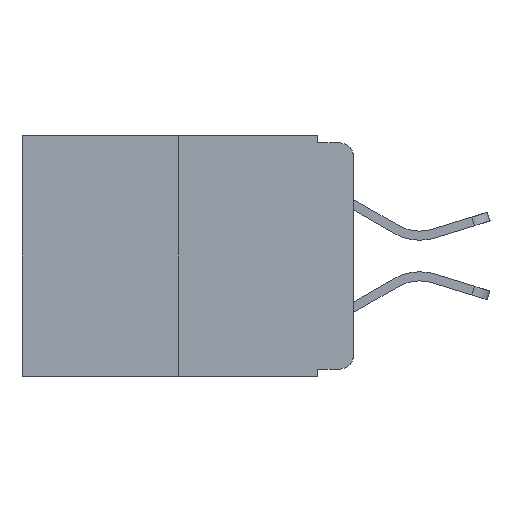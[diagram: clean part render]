
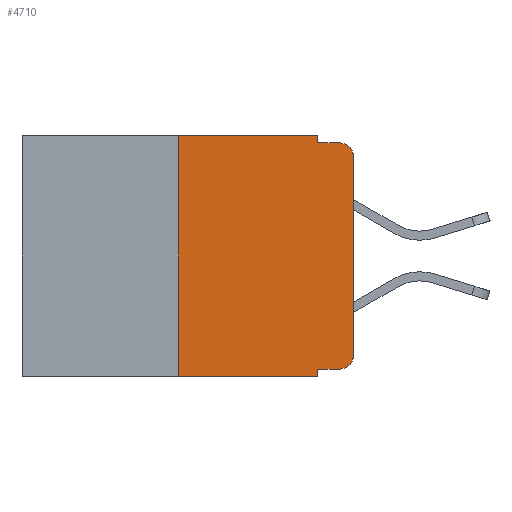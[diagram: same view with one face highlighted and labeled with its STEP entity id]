
A CAD part, left-side view. The second image highlights one B-rep face of the part: STEP entity #4710.
In plain terms, the highlighted planar face has unit normal (-1, 0, 0).
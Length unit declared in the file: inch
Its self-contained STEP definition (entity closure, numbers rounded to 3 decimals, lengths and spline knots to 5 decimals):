
#582 = EDGE_CURVE ( 'NONE', #12568, #9888, #10768, .T. ) ;
#737 = ORIENTED_EDGE ( 'NONE', *, *, #1405, .T. ) ;
#827 = CARTESIAN_POINT ( 'NONE',  ( 0., 0.051, -0.01 ) ) ;
#965 = CARTESIAN_POINT ( 'NONE',  ( 0., 0.473, -0.343 ) ) ;
#1026 = VERTEX_POINT ( 'NONE', #8154 ) ;
#1145 = AXIS2_PLACEMENT_3D ( 'NONE', #11117, #4868, #12154 ) ;
#1344 = DIRECTION ( 'NONE',  ( 0., -1., 0. ) ) ;
#1399 = CARTESIAN_POINT ( 'NONE',  ( 0., 0.051, -0.343 ) ) ;
#1405 = EDGE_CURVE ( 'NONE', #1777, #12568, #5124, .T. ) ;
#1473 = ORIENTED_EDGE ( 'NONE', *, *, #10100, .F. ) ;
#1503 = CARTESIAN_POINT ( 'NONE',  ( 0., 0.25, 0. ) ) ;
#1566 = DIRECTION ( 'NONE',  ( 0., 0., -1. ) ) ;
#1664 = ORIENTED_EDGE ( 'NONE', *, *, #2156, .F. ) ;
#1777 = VERTEX_POINT ( 'NONE', #2124 ) ;
#1992 = LINE ( 'NONE', #965, #12823 ) ;
#2124 = CARTESIAN_POINT ( 'NONE',  ( 0., 0.051, -0.333 ) ) ;
#2156 = EDGE_CURVE ( 'NONE', #1777, #13808, #5975, .T. ) ;
#2220 = CARTESIAN_POINT ( 'NONE',  ( 0., 0.02, -0.03 ) ) ;
#2394 = DIRECTION ( 'NONE',  ( 0., -1., 0. ) ) ;
#2566 = CARTESIAN_POINT ( 'NONE',  ( 0., 0.051, 0. ) ) ;
#2843 = EDGE_CURVE ( 'NONE', #7511, #9590, #5285, .T. ) ;
#3279 = DIRECTION ( 'NONE',  ( 0., 0., -1. ) ) ;
#3535 = VECTOR ( 'NONE', #8475, 39.37008 ) ;
#3605 = EDGE_CURVE ( 'NONE', #10144, #8338, #6113, .T. ) ;
#3803 = AXIS2_PLACEMENT_3D ( 'NONE', #2220, #9687, #3279 ) ;
#3881 = ORIENTED_EDGE ( 'NONE', *, *, #582, .T. ) ;
#3937 = DIRECTION ( 'NONE',  ( 0., 0., 1. ) ) ;
#4086 = VECTOR ( 'NONE', #10811, 39.37008 ) ;
#4267 = CARTESIAN_POINT ( 'NONE',  ( 0., 0.02, -0.313 ) ) ;
#4328 = EDGE_CURVE ( 'NONE', #8338, #11201, #6434, .T. ) ;
#4508 = CARTESIAN_POINT ( 'NONE',  ( 0., 0., 0. ) ) ;
#4710 = ADVANCED_FACE ( 'NONE', ( #13141 ), #11159, .F. ) ;
#4717 = ORIENTED_EDGE ( 'NONE', *, *, #2843, .F. ) ;
#4794 = VECTOR ( 'NONE', #1344, 39.37008 ) ;
#4868 = DIRECTION ( 'NONE',  ( 1., 0., 0. ) ) ;
#5043 = EDGE_CURVE ( 'NONE', #1026, #11201, #6889, .T. ) ;
#5124 = LINE ( 'NONE', #13704, #4794 ) ;
#5236 = CARTESIAN_POINT ( 'NONE',  ( 0., 0., -0.313 ) ) ;
#5285 = LINE ( 'NONE', #10262, #11184 ) ;
#5416 = CARTESIAN_POINT ( 'NONE',  ( 0., 0.02, -0.333 ) ) ;
#5627 = VECTOR ( 'NONE', #9076, 39.37008 ) ;
#5796 = EDGE_CURVE ( 'NONE', #9888, #1026, #12108, .T. ) ;
#5975 = LINE ( 'NONE', #10105, #5627 ) ;
#6113 = LINE ( 'NONE', #9641, #7603 ) ;
#6253 = LINE ( 'NONE', #8807, #11770 ) ;
#6434 = LINE ( 'NONE', #827, #3535 ) ;
#6889 = CIRCLE ( 'NONE', #3803, 0.02 ) ;
#7459 = CARTESIAN_POINT ( 'NONE',  ( 0., 0.02, -0.01 ) ) ;
#7511 = VERTEX_POINT ( 'NONE', #11187 ) ;
#7603 = VECTOR ( 'NONE', #11687, 39.37008 ) ;
#8154 = CARTESIAN_POINT ( 'NONE',  ( 0., 0., -0.03 ) ) ;
#8338 = VERTEX_POINT ( 'NONE', #8478 ) ;
#8475 = DIRECTION ( 'NONE',  ( 0., -1., 0. ) ) ;
#8478 = CARTESIAN_POINT ( 'NONE',  ( 0., 0.051, -0.01 ) ) ;
#8567 = EDGE_LOOP ( 'NONE', ( #10630, #11118, #8699, #9026, #1473, #4717, #11279, #1664, #737, #3881 ) ) ;
#8699 = ORIENTED_EDGE ( 'NONE', *, *, #4328, .F. ) ;
#8807 = CARTESIAN_POINT ( 'NONE',  ( 0., 0.473, 0. ) ) ;
#9026 = ORIENTED_EDGE ( 'NONE', *, *, #3605, .F. ) ;
#9076 = DIRECTION ( 'NONE',  ( 0., 0., -1. ) ) ;
#9590 = VERTEX_POINT ( 'NONE', #1503 ) ;
#9592 = DIRECTION ( 'NONE',  ( 0., -1., 0. ) ) ;
#9641 = CARTESIAN_POINT ( 'NONE',  ( 0., 0.051, 0. ) ) ;
#9687 = DIRECTION ( 'NONE',  ( -1., 0., 0. ) ) ;
#9888 = VERTEX_POINT ( 'NONE', #5236 ) ;
#9931 = EDGE_CURVE ( 'NONE', #7511, #13808, #1992, .T. ) ;
#10100 = EDGE_CURVE ( 'NONE', #9590, #10144, #6253, .T. ) ;
#10105 = CARTESIAN_POINT ( 'NONE',  ( 0., 0.051, 0. ) ) ;
#10144 = VERTEX_POINT ( 'NONE', #2566 ) ;
#10262 = CARTESIAN_POINT ( 'NONE',  ( 0., 0.25, 0. ) ) ;
#10630 = ORIENTED_EDGE ( 'NONE', *, *, #5796, .T. ) ;
#10768 = CIRCLE ( 'NONE', #11102, 0.02 ) ;
#10811 = DIRECTION ( 'NONE',  ( 0., 0., 1. ) ) ;
#10915 = DIRECTION ( 'NONE',  ( -1., 0., 0. ) ) ;
#11102 = AXIS2_PLACEMENT_3D ( 'NONE', #4267, #10915, #1566 ) ;
#11117 = CARTESIAN_POINT ( 'NONE',  ( 0., 0.473, 0. ) ) ;
#11118 = ORIENTED_EDGE ( 'NONE', *, *, #5043, .T. ) ;
#11159 = PLANE ( 'NONE',  #1145 ) ;
#11184 = VECTOR ( 'NONE', #3937, 39.37008 ) ;
#11187 = CARTESIAN_POINT ( 'NONE',  ( 0., 0.25, -0.343 ) ) ;
#11201 = VERTEX_POINT ( 'NONE', #7459 ) ;
#11279 = ORIENTED_EDGE ( 'NONE', *, *, #9931, .T. ) ;
#11687 = DIRECTION ( 'NONE',  ( 0., 0., -1. ) ) ;
#11770 = VECTOR ( 'NONE', #2394, 39.37008 ) ;
#12108 = LINE ( 'NONE', #4508, #4086 ) ;
#12154 = DIRECTION ( 'NONE',  ( 0., 0., -1. ) ) ;
#12568 = VERTEX_POINT ( 'NONE', #5416 ) ;
#12823 = VECTOR ( 'NONE', #9592, 39.37008 ) ;
#13141 = FACE_OUTER_BOUND ( 'NONE', #8567, .T. ) ;
#13704 = CARTESIAN_POINT ( 'NONE',  ( 0., 0.051, -0.333 ) ) ;
#13808 = VERTEX_POINT ( 'NONE', #1399 ) ;
